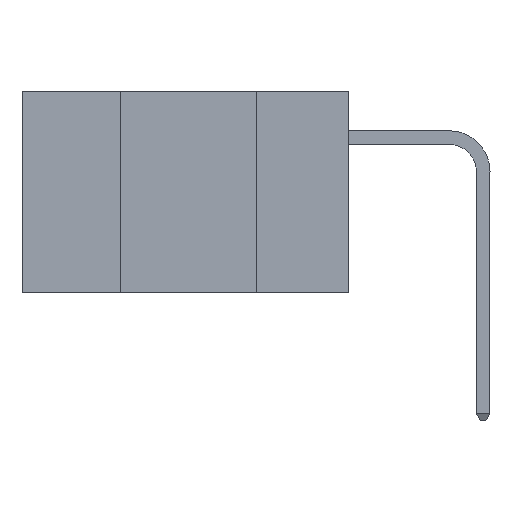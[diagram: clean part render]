
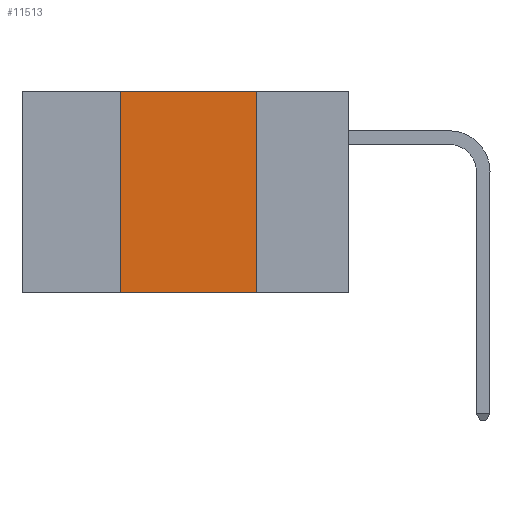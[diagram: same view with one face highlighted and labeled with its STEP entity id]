
A CAD part, left-side view. The second image highlights one B-rep face of the part: STEP entity #11513.
In plain terms, the highlighted planar face has unit normal (-1, 0, 0).
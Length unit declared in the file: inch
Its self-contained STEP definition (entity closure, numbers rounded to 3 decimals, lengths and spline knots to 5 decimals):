
#678 = VERTEX_POINT ( 'NONE', #5627 ) ;
#1242 = VERTEX_POINT ( 'NONE', #17421 ) ;
#2216 = EDGE_CURVE ( 'NONE', #1242, #17327, #19231, .T. ) ;
#2956 = EDGE_LOOP ( 'NONE', ( #19648, #10239, #14724, #18722 ) ) ;
#3244 = VECTOR ( 'NONE', #11470, 39.37008 ) ;
#4263 = EDGE_CURVE ( 'NONE', #1242, #15389, #19477, .T. ) ;
#5627 = CARTESIAN_POINT ( 'NONE',  ( 0., 0.17, 0. ) ) ;
#5775 = DIRECTION ( 'NONE',  ( 0., 0., -1. ) ) ;
#5903 = CARTESIAN_POINT ( 'NONE',  ( 0., 0.17, 0. ) ) ;
#8523 = DIRECTION ( 'NONE',  ( 0., -1., 0. ) ) ;
#8769 = EDGE_CURVE ( 'NONE', #678, #17327, #10543, .T. ) ;
#8853 = LINE ( 'NONE', #12465, #10320 ) ;
#10239 = ORIENTED_EDGE ( 'NONE', *, *, #19822, .F. ) ;
#10320 = VECTOR ( 'NONE', #18758, 39.37008 ) ;
#10543 = LINE ( 'NONE', #5903, #19532 ) ;
#10710 = AXIS2_PLACEMENT_3D ( 'NONE', #15969, #14393, #19132 ) ;
#11470 = DIRECTION ( 'NONE',  ( 0., 0., 1. ) ) ;
#11513 = ADVANCED_FACE ( 'NONE', ( #17323 ), #17526, .F. ) ;
#12465 = CARTESIAN_POINT ( 'NONE',  ( 0., 0.6, 0. ) ) ;
#14393 = DIRECTION ( 'NONE',  ( 1., 0., 0. ) ) ;
#14611 = CARTESIAN_POINT ( 'NONE',  ( 0., 0.42, 0. ) ) ;
#14724 = ORIENTED_EDGE ( 'NONE', *, *, #4263, .F. ) ;
#15132 = VECTOR ( 'NONE', #8523, 39.37008 ) ;
#15389 = VERTEX_POINT ( 'NONE', #14611 ) ;
#15419 = CARTESIAN_POINT ( 'NONE',  ( 0., 0.17, -0.37 ) ) ;
#15969 = CARTESIAN_POINT ( 'NONE',  ( 0., 0.6, 0. ) ) ;
#17323 = FACE_OUTER_BOUND ( 'NONE', #2956, .T. ) ;
#17327 = VERTEX_POINT ( 'NONE', #15419 ) ;
#17421 = CARTESIAN_POINT ( 'NONE',  ( 0., 0.42, -0.37 ) ) ;
#17526 = PLANE ( 'NONE',  #10710 ) ;
#17950 = CARTESIAN_POINT ( 'NONE',  ( 0., 0.42, 0. ) ) ;
#18707 = CARTESIAN_POINT ( 'NONE',  ( 0., 0.6, -0.37 ) ) ;
#18722 = ORIENTED_EDGE ( 'NONE', *, *, #2216, .T. ) ;
#18758 = DIRECTION ( 'NONE',  ( 0., -1., 0. ) ) ;
#19132 = DIRECTION ( 'NONE',  ( 0., 0., -1. ) ) ;
#19231 = LINE ( 'NONE', #18707, #15132 ) ;
#19477 = LINE ( 'NONE', #17950, #3244 ) ;
#19532 = VECTOR ( 'NONE', #5775, 39.37008 ) ;
#19648 = ORIENTED_EDGE ( 'NONE', *, *, #8769, .F. ) ;
#19822 = EDGE_CURVE ( 'NONE', #15389, #678, #8853, .T. ) ;
